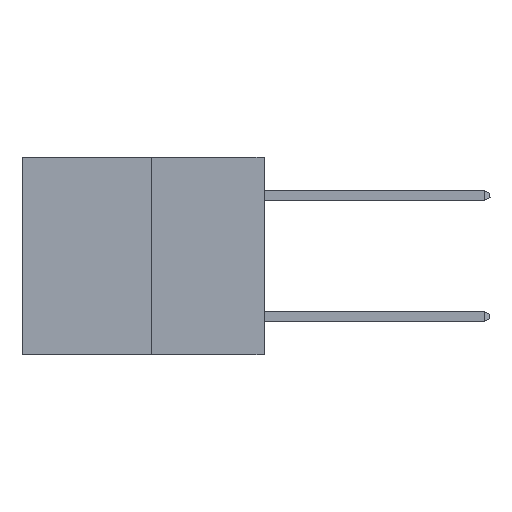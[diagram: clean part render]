
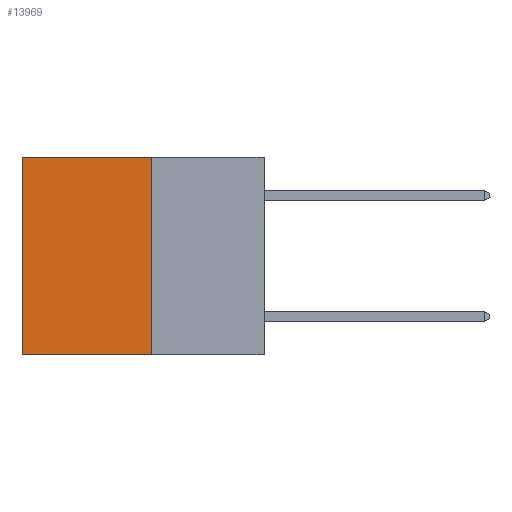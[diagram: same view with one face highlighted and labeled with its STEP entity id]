
A CAD part, left-side view. The second image highlights one B-rep face of the part: STEP entity #13969.
In plain terms, the highlighted planar face has unit normal (-1, 0, 0).
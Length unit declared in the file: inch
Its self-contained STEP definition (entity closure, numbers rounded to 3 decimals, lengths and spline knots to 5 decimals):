
#9 = VERTEX_POINT ( 'NONE', #1739 ) ;
#426 = VERTEX_POINT ( 'NONE', #8382 ) ;
#558 = EDGE_LOOP ( 'NONE', ( #14401, #9175, #24693, #13767 ) ) ;
#1739 = CARTESIAN_POINT ( 'NONE',  ( 0.3165, 0.6, 0. ) ) ;
#1913 = DIRECTION ( 'NONE',  ( 0., 1., 0. ) ) ;
#2508 = CARTESIAN_POINT ( 'NONE',  ( 0.3165, 0.28, -0.49 ) ) ;
#3555 = VECTOR ( 'NONE', #21942, 39.37008 ) ;
#3760 = EDGE_CURVE ( 'NONE', #426, #21514, #12784, .T. ) ;
#4213 = DIRECTION ( 'NONE',  ( 1., 0., 0. ) ) ;
#4561 = CARTESIAN_POINT ( 'NONE',  ( 0.3165, 0.28, -0.49 ) ) ;
#7260 = EDGE_CURVE ( 'NONE', #9, #22765, #8868, .T. ) ;
#7459 = VECTOR ( 'NONE', #7952, 39.37008 ) ;
#7952 = DIRECTION ( 'NONE',  ( 0., 0., -1. ) ) ;
#8382 = CARTESIAN_POINT ( 'NONE',  ( 0.3165, 0.28, 0. ) ) ;
#8868 = LINE ( 'NONE', #21519, #3555 ) ;
#9030 = DIRECTION ( 'NONE',  ( 0., 1., 0. ) ) ;
#9175 = ORIENTED_EDGE ( 'NONE', *, *, #20179, .F. ) ;
#9989 = VECTOR ( 'NONE', #1913, 39.37008 ) ;
#10134 = DIRECTION ( 'NONE',  ( 0., 0., -1. ) ) ;
#11040 = LINE ( 'NONE', #17365, #20494 ) ;
#12784 = LINE ( 'NONE', #22013, #7459 ) ;
#13767 = ORIENTED_EDGE ( 'NONE', *, *, #15544, .T. ) ;
#13969 = ADVANCED_FACE ( 'NONE', ( #24696 ), #16351, .F. ) ;
#14401 = ORIENTED_EDGE ( 'NONE', *, *, #7260, .T. ) ;
#15544 = EDGE_CURVE ( 'NONE', #426, #9, #11040, .T. ) ;
#15826 = CARTESIAN_POINT ( 'NONE',  ( 0.3165, 0.28, -0.49 ) ) ;
#16351 = PLANE ( 'NONE',  #25950 ) ;
#17365 = CARTESIAN_POINT ( 'NONE',  ( 0.3165, 0.28, 0. ) ) ;
#17707 = CARTESIAN_POINT ( 'NONE',  ( 0.3165, 0.6, -0.49 ) ) ;
#20179 = EDGE_CURVE ( 'NONE', #21514, #22765, #23525, .T. ) ;
#20494 = VECTOR ( 'NONE', #9030, 39.37008 ) ;
#21514 = VERTEX_POINT ( 'NONE', #2508 ) ;
#21519 = CARTESIAN_POINT ( 'NONE',  ( 0.3165, 0.6, -0.49 ) ) ;
#21942 = DIRECTION ( 'NONE',  ( 0., 0., -1. ) ) ;
#22013 = CARTESIAN_POINT ( 'NONE',  ( 0.3165, 0.28, -0.49 ) ) ;
#22765 = VERTEX_POINT ( 'NONE', #17707 ) ;
#23525 = LINE ( 'NONE', #15826, #9989 ) ;
#24693 = ORIENTED_EDGE ( 'NONE', *, *, #3760, .F. ) ;
#24696 = FACE_OUTER_BOUND ( 'NONE', #558, .T. ) ;
#25950 = AXIS2_PLACEMENT_3D ( 'NONE', #4561, #4213, #10134 ) ;
